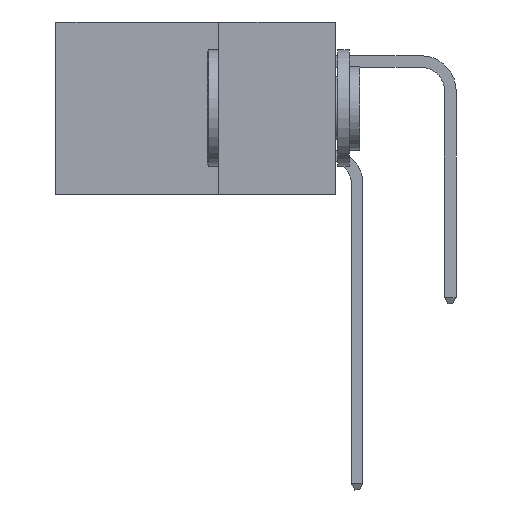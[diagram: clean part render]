
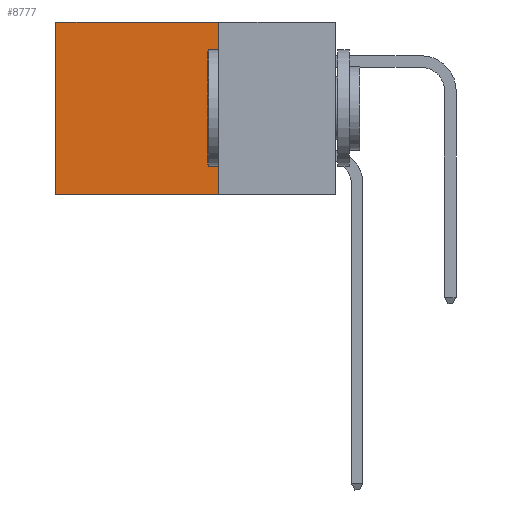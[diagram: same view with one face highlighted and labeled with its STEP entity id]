
A CAD part, left-side view. The second image highlights one B-rep face of the part: STEP entity #8777.
In plain terms, the highlighted planar face has unit normal (-1, 0, 0).
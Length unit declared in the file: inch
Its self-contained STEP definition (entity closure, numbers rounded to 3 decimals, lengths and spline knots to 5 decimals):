
#84 = EDGE_CURVE ( 'NONE', #2696, #20195, #6097, .T. ) ;
#94 = EDGE_CURVE ( 'NONE', #2696, #1621, #7861, .T. ) ;
#210 = CARTESIAN_POINT ( 'NONE',  ( 0.2875, 0.6, 0. ) ) ;
#1621 = VERTEX_POINT ( 'NONE', #15389 ) ;
#1876 = DIRECTION ( 'NONE',  ( 0., 0., -1. ) ) ;
#2447 = LINE ( 'NONE', #210, #4231 ) ;
#2696 = VERTEX_POINT ( 'NONE', #17181 ) ;
#3433 = VERTEX_POINT ( 'NONE', #19909 ) ;
#3576 = VECTOR ( 'NONE', #12467, 39.37008 ) ;
#4231 = VECTOR ( 'NONE', #1876, 39.37008 ) ;
#5093 = VECTOR ( 'NONE', #20550, 39.37008 ) ;
#5896 = EDGE_LOOP ( 'NONE', ( #7134, #7862, #15829, #19222 ) ) ;
#5963 = CARTESIAN_POINT ( 'NONE',  ( 0.2875, 0.25, 0. ) ) ;
#6002 = PLANE ( 'NONE',  #14139 ) ;
#6097 = LINE ( 'NONE', #18929, #5093 ) ;
#7134 = ORIENTED_EDGE ( 'NONE', *, *, #10618, .T. ) ;
#7861 = LINE ( 'NONE', #5963, #3576 ) ;
#7862 = ORIENTED_EDGE ( 'NONE', *, *, #8733, .F. ) ;
#8461 = CARTESIAN_POINT ( 'NONE',  ( 0.2875, 0.25, -0.37 ) ) ;
#8733 = EDGE_CURVE ( 'NONE', #20195, #3433, #20527, .T. ) ;
#8777 = ADVANCED_FACE ( 'NONE', ( #17995 ), #6002, .F. ) ;
#9154 = CARTESIAN_POINT ( 'NONE',  ( 0.2875, 0.25, -0.37 ) ) ;
#9320 = CARTESIAN_POINT ( 'NONE',  ( 0.2875, 0.25, 0. ) ) ;
#9363 = VECTOR ( 'NONE', #19805, 39.37008 ) ;
#10618 = EDGE_CURVE ( 'NONE', #1621, #3433, #2447, .T. ) ;
#10824 = DIRECTION ( 'NONE',  ( 0., 0., -1. ) ) ;
#12467 = DIRECTION ( 'NONE',  ( 0., 1., 0. ) ) ;
#14139 = AXIS2_PLACEMENT_3D ( 'NONE', #9320, #20586, #10824 ) ;
#15389 = CARTESIAN_POINT ( 'NONE',  ( 0.2875, 0.6, 0. ) ) ;
#15829 = ORIENTED_EDGE ( 'NONE', *, *, #84, .F. ) ;
#17181 = CARTESIAN_POINT ( 'NONE',  ( 0.2875, 0.25, 0. ) ) ;
#17995 = FACE_OUTER_BOUND ( 'NONE', #5896, .T. ) ;
#18929 = CARTESIAN_POINT ( 'NONE',  ( 0.2875, 0.25, 0. ) ) ;
#19222 = ORIENTED_EDGE ( 'NONE', *, *, #94, .T. ) ;
#19805 = DIRECTION ( 'NONE',  ( 0., 1., 0. ) ) ;
#19909 = CARTESIAN_POINT ( 'NONE',  ( 0.2875, 0.6, -0.37 ) ) ;
#20195 = VERTEX_POINT ( 'NONE', #9154 ) ;
#20527 = LINE ( 'NONE', #8461, #9363 ) ;
#20550 = DIRECTION ( 'NONE',  ( 0., 0., -1. ) ) ;
#20586 = DIRECTION ( 'NONE',  ( 1., 0., 0. ) ) ;
